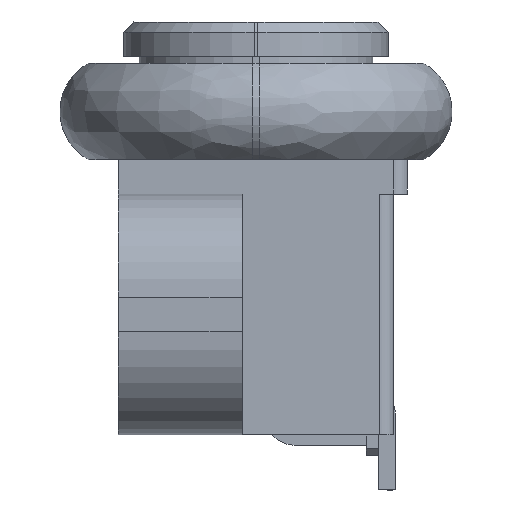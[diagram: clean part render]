
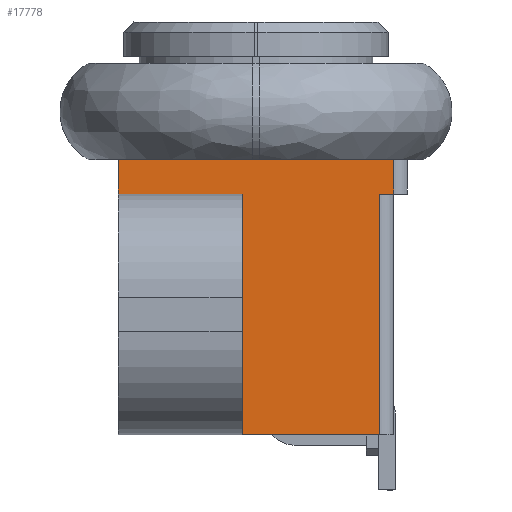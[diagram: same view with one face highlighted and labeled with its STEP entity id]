
A CAD part, left-side view. The second image highlights one B-rep face of the part: STEP entity #17778.
In plain terms, the highlighted face is planar.
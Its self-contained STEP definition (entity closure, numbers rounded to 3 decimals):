
#1094 = AXIS2_PLACEMENT_3D ( 'NONE', #2233, #18496, #10484 ) ;
#2233 = CARTESIAN_POINT ( 'NONE',  ( -1.88, -1.83, 5. ) ) ;
#2365 = DIRECTION ( 'NONE',  ( 0., -1., 0. ) ) ;
#2569 = DIRECTION ( 'NONE',  ( 1., 0., 0. ) ) ;
#2731 = EDGE_CURVE ( 'NONE', #7978, #12156, #19655, .T. ) ;
#2794 = EDGE_CURVE ( 'NONE', #12156, #18994, #6683, .T. ) ;
#3381 = DIRECTION ( 'NONE',  ( 1., 0., 0. ) ) ;
#3446 = ORIENTED_EDGE ( 'NONE', *, *, #2794, .T. ) ;
#4498 = CARTESIAN_POINT ( 'NONE',  ( -1.8, 2.25, 5. ) ) ;
#5349 = CARTESIAN_POINT ( 'NONE',  ( 2., -1.75, 5. ) ) ;
#5928 = VERTEX_POINT ( 'NONE', #13578 ) ;
#6356 = DIRECTION ( 'NONE',  ( 1., 0., 0. ) ) ;
#6591 = VERTEX_POINT ( 'NONE', #4498 ) ;
#6683 = LINE ( 'NONE', #8592, #10761 ) ;
#7031 = LINE ( 'NONE', #8734, #13089 ) ;
#7271 = VERTEX_POINT ( 'NONE', #13050 ) ;
#7678 = CARTESIAN_POINT ( 'NONE',  ( -1.8, 1.75, 5. ) ) ;
#7978 = VERTEX_POINT ( 'NONE', #7678 ) ;
#8247 = LINE ( 'NONE', #10045, #18042 ) ;
#8402 = CARTESIAN_POINT ( 'NONE',  ( -1.8, 0.25, 5. ) ) ;
#8519 = ORIENTED_EDGE ( 'NONE', *, *, #13526, .F. ) ;
#8592 = CARTESIAN_POINT ( 'NONE',  ( 0., 0., 5. ) ) ;
#8734 = CARTESIAN_POINT ( 'NONE',  ( 2., 0.25, 5. ) ) ;
#9168 = VECTOR ( 'NONE', #9995, 1000. ) ;
#9413 = EDGE_CURVE ( 'NONE', #10832, #19104, #7031, .T. ) ;
#9914 = CARTESIAN_POINT ( 'NONE',  ( 0., -1.75, 5. ) ) ;
#9957 = VECTOR ( 'NONE', #2569, 1000. ) ;
#9995 = DIRECTION ( 'NONE',  ( 0., 1., 0. ) ) ;
#10045 = CARTESIAN_POINT ( 'NONE',  ( 2.2, 0.25, 5. ) ) ;
#10484 = DIRECTION ( 'NONE',  ( 1., 0., 0. ) ) ;
#10761 = VECTOR ( 'NONE', #15089, 1000. ) ;
#10832 = VERTEX_POINT ( 'NONE', #19669 ) ;
#10881 = ORIENTED_EDGE ( 'NONE', *, *, #17318, .T. ) ;
#11441 = LINE ( 'NONE', #12939, #11939 ) ;
#11642 = DIRECTION ( 'NONE',  ( 0., -1., 0. ) ) ;
#11663 = LINE ( 'NONE', #14661, #13205 ) ;
#11939 = VECTOR ( 'NONE', #3381, 1000. ) ;
#11995 = PLANE ( 'NONE',  #1094 ) ;
#12156 = VERTEX_POINT ( 'NONE', #12632 ) ;
#12342 = EDGE_CURVE ( 'NONE', #6591, #5928, #11663, .T. ) ;
#12477 = VECTOR ( 'NONE', #14987, 1000. ) ;
#12632 = CARTESIAN_POINT ( 'NONE',  ( 0., 1.75, 5. ) ) ;
#12939 = CARTESIAN_POINT ( 'NONE',  ( 0.2, -1.75, 5. ) ) ;
#13001 = ORIENTED_EDGE ( 'NONE', *, *, #18030, .T. ) ;
#13050 = CARTESIAN_POINT ( 'NONE',  ( 2.2, 1.75, 5. ) ) ;
#13089 = VECTOR ( 'NONE', #2365, 1000. ) ;
#13205 = VECTOR ( 'NONE', #6356, 1000. ) ;
#13406 = LINE ( 'NONE', #8402, #9168 ) ;
#13434 = EDGE_LOOP ( 'NONE', ( #18108, #8519, #14129, #3446, #13001, #14968, #10881, #19564 ) ) ;
#13526 = EDGE_CURVE ( 'NONE', #7978, #6591, #13406, .T. ) ;
#13578 = CARTESIAN_POINT ( 'NONE',  ( 2.2, 2.25, 5. ) ) ;
#14129 = ORIENTED_EDGE ( 'NONE', *, *, #2731, .T. ) ;
#14661 = CARTESIAN_POINT ( 'NONE',  ( 0.2, 2.25, 5. ) ) ;
#14879 = CARTESIAN_POINT ( 'NONE',  ( -0.9, 1.75, 5. ) ) ;
#14968 = ORIENTED_EDGE ( 'NONE', *, *, #9413, .F. ) ;
#14987 = DIRECTION ( 'NONE',  ( 1., 0., 0. ) ) ;
#15089 = DIRECTION ( 'NONE',  ( 0., -1., 0. ) ) ;
#15092 = FACE_OUTER_BOUND ( 'NONE', #13434, .T. ) ;
#15138 = EDGE_CURVE ( 'NONE', #5928, #7271, #8247, .T. ) ;
#17318 = EDGE_CURVE ( 'NONE', #10832, #7271, #20307, .T. ) ;
#17778 = ADVANCED_FACE ( 'NONE', ( #15092 ), #11995, .T. ) ;
#18030 = EDGE_CURVE ( 'NONE', #18994, #19104, #11441, .T. ) ;
#18042 = VECTOR ( 'NONE', #11642, 1000. ) ;
#18108 = ORIENTED_EDGE ( 'NONE', *, *, #12342, .F. ) ;
#18496 = DIRECTION ( 'NONE',  ( 0., 0., 1. ) ) ;
#18615 = CARTESIAN_POINT ( 'NONE',  ( 2.2, 1.75, 5. ) ) ;
#18994 = VERTEX_POINT ( 'NONE', #9914 ) ;
#19104 = VERTEX_POINT ( 'NONE', #5349 ) ;
#19564 = ORIENTED_EDGE ( 'NONE', *, *, #15138, .F. ) ;
#19655 = LINE ( 'NONE', #14879, #12477 ) ;
#19669 = CARTESIAN_POINT ( 'NONE',  ( 2., 1.75, 5. ) ) ;
#20307 = LINE ( 'NONE', #18615, #9957 ) ;
